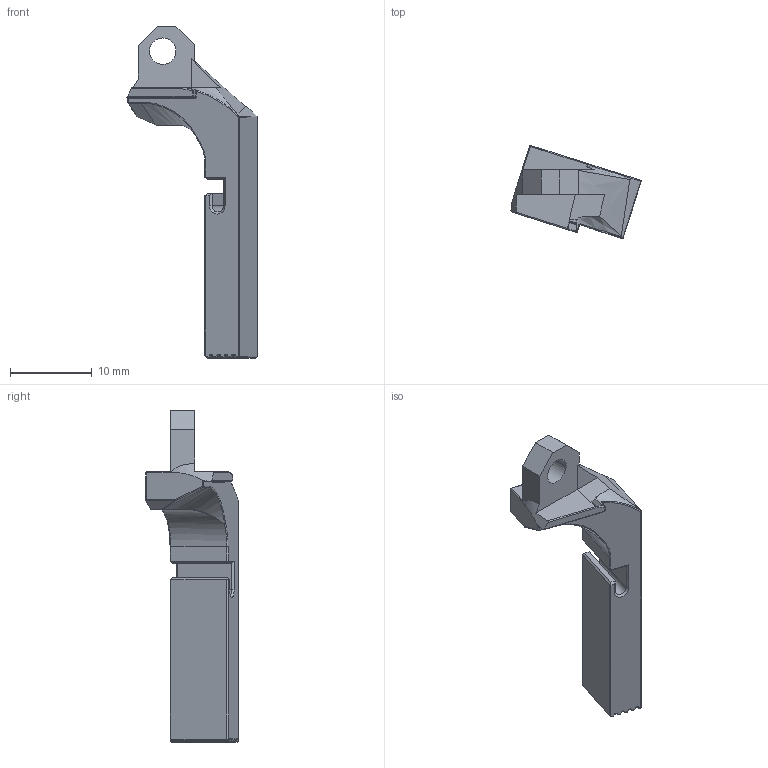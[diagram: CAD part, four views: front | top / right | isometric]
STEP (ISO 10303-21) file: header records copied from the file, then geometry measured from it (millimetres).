
FILE_DESCRIPTION(/* description */ (''),/* implementation_level */ '2;1');
FILE_NAME(/* name */ 'solo mag catch.step',/* time_stamp */ '2021-05-31T19:22:20-06:00',/* author */ (''),/* organization */ (''),/* preprocessor_version */ 'ST-DEVELOPER v18.1',/* originating_system */ 'Autodesk Translation Framework v10.9.0.1377',/* authorisation */ '');
FILE_SCHEMA (('AUTOMOTIVE_DESIGN { 1 0 10303 214 3 1 1 }'));
Length unit declared in the file: millimetre
Products named in the file (1): solo mag catch
Bounding box: 15.96 x 11.36 x 40.73 mm (x, y, z)
Volume: 1446.7 mm3; surface area: 1236.6 mm2
Topology: 1 solids, 1 shells, 169 faces, 407 edges, 240 vertices
Faces by surface type: cylinder 65, plane 49, bspline 28, torus 14, sphere 11, cone 2
Full cylindrical faces by diameter (mm): 3.25 x1
Entity records: 9962 total; most frequent: CARTESIAN_POINT 6080, ORIENTED_EDGE 814, DIRECTION 812, EDGE_CURVE 407, AXIS2_PLACEMENT_3D 313, VERTEX_POINT 240, LINE 186, VECTOR 186
